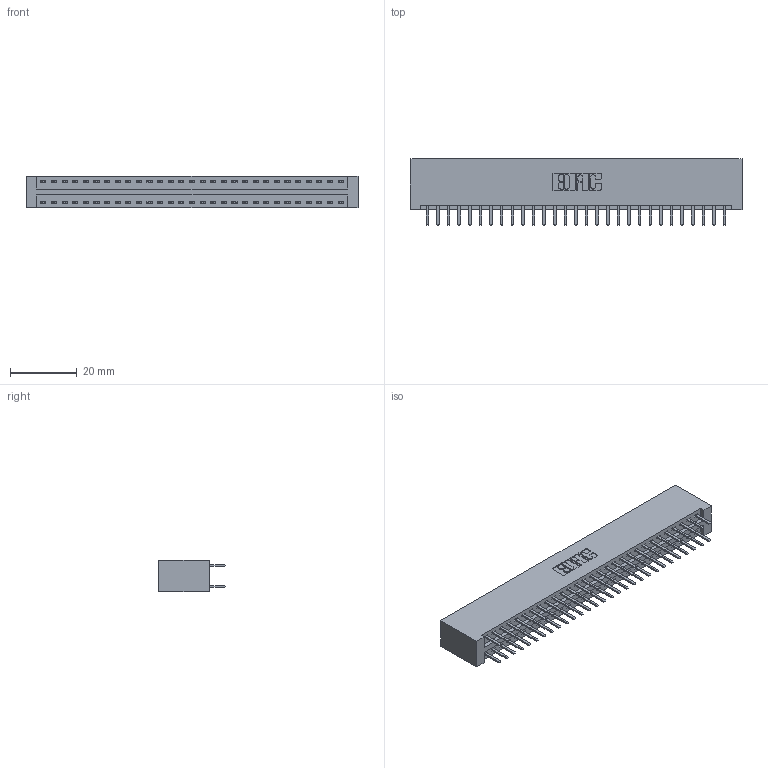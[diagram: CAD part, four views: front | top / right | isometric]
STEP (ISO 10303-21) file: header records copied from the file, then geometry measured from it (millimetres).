
FILE_DESCRIPTION (( 'STEP AP203' ), '1' );
FILE_NAME ('396-058-520-201.STEP', '2019-10-30T15:55:43', ( '' ), ( '' ), 'SwSTEP 2.0', 'SolidWorks 2016', '' );
FILE_SCHEMA (( 'CONFIG_CONTROL_DESIGN' ));
Length unit declared in the file: inch
Products named in the file (3): 396-058-520-201; 345-292-001_345-293-120; 346 Part_No Mounting Lugs
Assembly tree (59 placements, depth 2):
  396-058-520-201
    346 Part_No Mounting Lugs
    345-292-001_345-293-120  x58
Bounding box: 99.31 x 20.02 x 9.4 mm (x, y, z)
Volume: 10131.2 mm3; surface area: 13825.1 mm2
Topology: 59 solids, 59 shells, 3362 faces, 9759 edges, 6350 vertices
Faces by surface type: plane 2218, cylinder 1144
Entity records: 20513 total; most frequent: CARTESIAN_POINT 3408, ORIENTED_EDGE 3330, DIRECTION 3037, EDGE_CURVE 1665, VECTOR 1421, LINE 1421, VERTEX_POINT 1106, AXIS2_PLACEMENT_3D 808
